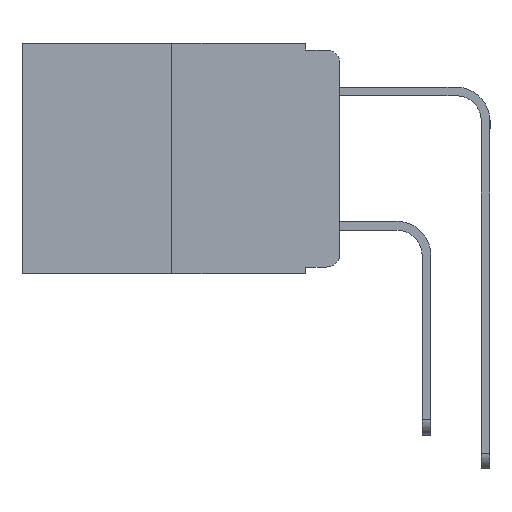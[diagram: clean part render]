
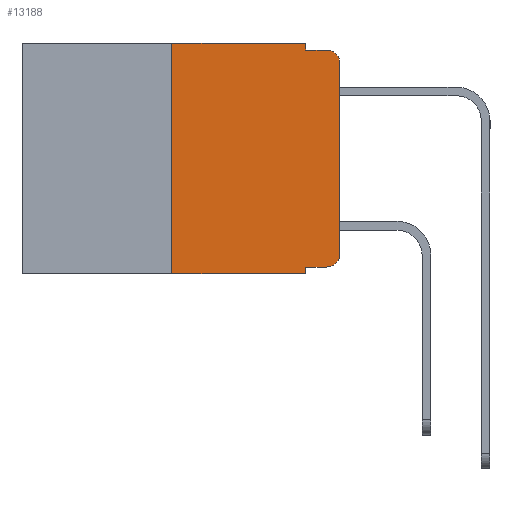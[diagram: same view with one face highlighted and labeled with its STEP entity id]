
A CAD part, left-side view. The second image highlights one B-rep face of the part: STEP entity #13188.
In plain terms, the highlighted planar face has unit normal (-1, 0, 0).
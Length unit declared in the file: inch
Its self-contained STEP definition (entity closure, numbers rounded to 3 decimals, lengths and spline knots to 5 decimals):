
#915 = VECTOR ( 'NONE', #15238, 39.37008 ) ;
#1274 = ORIENTED_EDGE ( 'NONE', *, *, #5153, .F. ) ;
#1456 = LINE ( 'NONE', #14172, #9093 ) ;
#1556 = CARTESIAN_POINT ( 'NONE',  ( 0., 0.02, -0.313 ) ) ;
#1965 = AXIS2_PLACEMENT_3D ( 'NONE', #2011, #12267, #3656 ) ;
#2011 = CARTESIAN_POINT ( 'NONE',  ( 0., 0.473, 0. ) ) ;
#2173 = CARTESIAN_POINT ( 'NONE',  ( 0., 0.051, -0.333 ) ) ;
#2179 = CARTESIAN_POINT ( 'NONE',  ( 0., 0.051, -0.333 ) ) ;
#2307 = CARTESIAN_POINT ( 'NONE',  ( 0., 0.051, -0.01 ) ) ;
#2572 = CARTESIAN_POINT ( 'NONE',  ( 0., 0.02, -0.03 ) ) ;
#3234 = DIRECTION ( 'NONE',  ( 0., 0., -1. ) ) ;
#3410 = ORIENTED_EDGE ( 'NONE', *, *, #7142, .F. ) ;
#3656 = DIRECTION ( 'NONE',  ( 0., 0., -1. ) ) ;
#3693 = CARTESIAN_POINT ( 'NONE',  ( 0., 0.051, 0. ) ) ;
#3934 = CARTESIAN_POINT ( 'NONE',  ( 0., 0.25, 0. ) ) ;
#3960 = ORIENTED_EDGE ( 'NONE', *, *, #18362, .T. ) ;
#4087 = DIRECTION ( 'NONE',  ( 0., 0., -1. ) ) ;
#4110 = ORIENTED_EDGE ( 'NONE', *, *, #8115, .T. ) ;
#4131 = EDGE_CURVE ( 'NONE', #12711, #8332, #1456, .T. ) ;
#4146 = DIRECTION ( 'NONE',  ( 0., 0., -1. ) ) ;
#4235 = EDGE_LOOP ( 'NONE', ( #4364, #4110, #3410, #11108, #8506, #1274, #11341, #5736, #4907, #3960 ) ) ;
#4332 = VERTEX_POINT ( 'NONE', #13240 ) ;
#4364 = ORIENTED_EDGE ( 'NONE', *, *, #9076, .T. ) ;
#4419 = CARTESIAN_POINT ( 'NONE',  ( 0., 0., -0.03 ) ) ;
#4754 = VERTEX_POINT ( 'NONE', #4419 ) ;
#4787 = CARTESIAN_POINT ( 'NONE',  ( 0., 0., 0. ) ) ;
#4907 = ORIENTED_EDGE ( 'NONE', *, *, #17524, .T. ) ;
#5153 = EDGE_CURVE ( 'NONE', #14350, #12397, #16653, .T. ) ;
#5291 = VECTOR ( 'NONE', #14693, 39.37008 ) ;
#5736 = ORIENTED_EDGE ( 'NONE', *, *, #4131, .F. ) ;
#6054 = CARTESIAN_POINT ( 'NONE',  ( 0., 0.051, -0.343 ) ) ;
#6157 = EDGE_CURVE ( 'NONE', #4332, #14015, #9848, .T. ) ;
#6280 = CARTESIAN_POINT ( 'NONE',  ( 0., 0.25, 0. ) ) ;
#6813 = CARTESIAN_POINT ( 'NONE',  ( 0., 0.02, -0.333 ) ) ;
#6815 = DIRECTION ( 'NONE',  ( 0., -1., 0. ) ) ;
#7142 = EDGE_CURVE ( 'NONE', #14015, #10311, #8480, .T. ) ;
#7636 = CIRCLE ( 'NONE', #13260, 0.02 ) ;
#7679 = VECTOR ( 'NONE', #6815, 39.37008 ) ;
#8115 = EDGE_CURVE ( 'NONE', #4754, #10311, #7636, .T. ) ;
#8332 = VERTEX_POINT ( 'NONE', #6054 ) ;
#8480 = LINE ( 'NONE', #2307, #15357 ) ;
#8506 = ORIENTED_EDGE ( 'NONE', *, *, #12671, .F. ) ;
#8983 = CARTESIAN_POINT ( 'NONE',  ( 0., 0.051, -0.01 ) ) ;
#8984 = VECTOR ( 'NONE', #4087, 39.37008 ) ;
#9037 = VECTOR ( 'NONE', #11203, 39.37008 ) ;
#9076 = EDGE_CURVE ( 'NONE', #15881, #4754, #15188, .T. ) ;
#9093 = VECTOR ( 'NONE', #15464, 39.37008 ) ;
#9538 = LINE ( 'NONE', #17743, #915 ) ;
#9848 = LINE ( 'NONE', #3693, #8984 ) ;
#10311 = VERTEX_POINT ( 'NONE', #12085 ) ;
#10898 = PLANE ( 'NONE',  #1965 ) ;
#11073 = CARTESIAN_POINT ( 'NONE',  ( 0., 0., -0.313 ) ) ;
#11108 = ORIENTED_EDGE ( 'NONE', *, *, #6157, .F. ) ;
#11203 = DIRECTION ( 'NONE',  ( 0., 0., 1. ) ) ;
#11341 = ORIENTED_EDGE ( 'NONE', *, *, #14544, .T. ) ;
#11378 = LINE ( 'NONE', #13837, #7679 ) ;
#11894 = DIRECTION ( 'NONE',  ( -1., 0., 0. ) ) ;
#11899 = AXIS2_PLACEMENT_3D ( 'NONE', #1556, #11894, #3234 ) ;
#12085 = CARTESIAN_POINT ( 'NONE',  ( 0., 0.02, -0.01 ) ) ;
#12267 = DIRECTION ( 'NONE',  ( 1., 0., 0. ) ) ;
#12397 = VERTEX_POINT ( 'NONE', #6280 ) ;
#12507 = DIRECTION ( 'NONE',  ( 0., -1., 0. ) ) ;
#12671 = EDGE_CURVE ( 'NONE', #12397, #4332, #9538, .T. ) ;
#12711 = VERTEX_POINT ( 'NONE', #2179 ) ;
#12713 = VERTEX_POINT ( 'NONE', #6813 ) ;
#12725 = DIRECTION ( 'NONE',  ( -1., 0., 0. ) ) ;
#13188 = ADVANCED_FACE ( 'NONE', ( #15482 ), #10898, .F. ) ;
#13240 = CARTESIAN_POINT ( 'NONE',  ( 0., 0.051, 0. ) ) ;
#13260 = AXIS2_PLACEMENT_3D ( 'NONE', #2572, #12725, #4146 ) ;
#13298 = CIRCLE ( 'NONE', #11899, 0.02 ) ;
#13837 = CARTESIAN_POINT ( 'NONE',  ( 0., 0.473, -0.343 ) ) ;
#14015 = VERTEX_POINT ( 'NONE', #8983 ) ;
#14172 = CARTESIAN_POINT ( 'NONE',  ( 0., 0.051, 0. ) ) ;
#14350 = VERTEX_POINT ( 'NONE', #16233 ) ;
#14544 = EDGE_CURVE ( 'NONE', #14350, #8332, #11378, .T. ) ;
#14693 = DIRECTION ( 'NONE',  ( 0., 0., 1. ) ) ;
#15160 = DIRECTION ( 'NONE',  ( 0., -1., 0. ) ) ;
#15188 = LINE ( 'NONE', #4787, #5291 ) ;
#15238 = DIRECTION ( 'NONE',  ( 0., -1., 0. ) ) ;
#15357 = VECTOR ( 'NONE', #12507, 39.37008 ) ;
#15464 = DIRECTION ( 'NONE',  ( 0., 0., -1. ) ) ;
#15482 = FACE_OUTER_BOUND ( 'NONE', #4235, .T. ) ;
#15881 = VERTEX_POINT ( 'NONE', #11073 ) ;
#16233 = CARTESIAN_POINT ( 'NONE',  ( 0., 0.25, -0.343 ) ) ;
#16418 = VECTOR ( 'NONE', #15160, 39.37008 ) ;
#16653 = LINE ( 'NONE', #3934, #9037 ) ;
#16798 = LINE ( 'NONE', #2173, #16418 ) ;
#17524 = EDGE_CURVE ( 'NONE', #12711, #12713, #16798, .T. ) ;
#17743 = CARTESIAN_POINT ( 'NONE',  ( 0., 0.473, 0. ) ) ;
#18362 = EDGE_CURVE ( 'NONE', #12713, #15881, #13298, .T. ) ;
